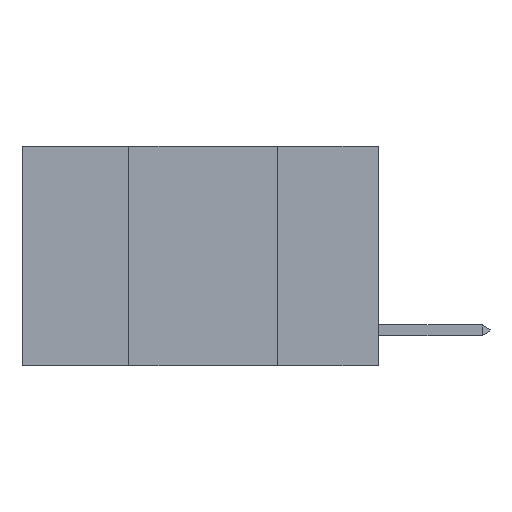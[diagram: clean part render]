
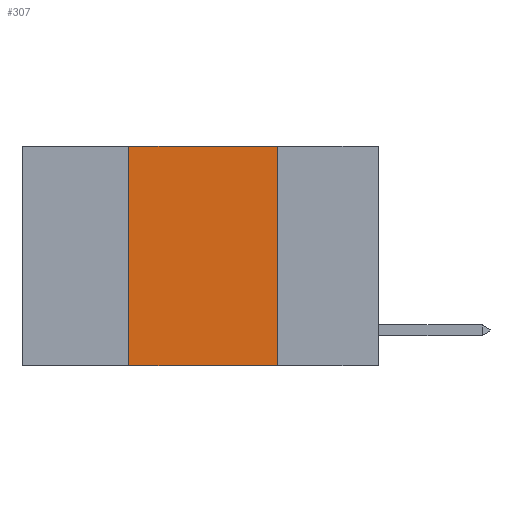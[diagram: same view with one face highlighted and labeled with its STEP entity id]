
A CAD part, left-side view. The second image highlights one B-rep face of the part: STEP entity #307.
In plain terms, the highlighted planar face has unit normal (-1, 0, 0).
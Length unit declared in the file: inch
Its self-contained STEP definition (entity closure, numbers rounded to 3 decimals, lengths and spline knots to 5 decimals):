
#183 = DIRECTION ( 'NONE',  ( 0., 0., 1. ) ) ;
#307 = ADVANCED_FACE ( 'NONE', ( #6110 ), #3378, .F. ) ;
#544 = DIRECTION ( 'NONE',  ( 0., 0., -1. ) ) ;
#657 = VERTEX_POINT ( 'NONE', #7695 ) ;
#913 = VERTEX_POINT ( 'NONE', #3167 ) ;
#953 = DIRECTION ( 'NONE',  ( 0., -1., 0. ) ) ;
#1651 = EDGE_CURVE ( 'NONE', #657, #3464, #7738, .T. ) ;
#1752 = LINE ( 'NONE', #4094, #5136 ) ;
#1923 = ORIENTED_EDGE ( 'NONE', *, *, #1651, .F. ) ;
#2455 = VECTOR ( 'NONE', #8177, 39.37008 ) ;
#2911 = ORIENTED_EDGE ( 'NONE', *, *, #6931, .F. ) ;
#3108 = CARTESIAN_POINT ( 'NONE',  ( 0., 0.42, 0. ) ) ;
#3167 = CARTESIAN_POINT ( 'NONE',  ( 0., 0.42, -0.37 ) ) ;
#3378 = PLANE ( 'NONE',  #3609 ) ;
#3464 = VERTEX_POINT ( 'NONE', #7201 ) ;
#3609 = AXIS2_PLACEMENT_3D ( 'NONE', #4952, #7891, #6412 ) ;
#3915 = CARTESIAN_POINT ( 'NONE',  ( 0., 0.17, -0.37 ) ) ;
#4050 = LINE ( 'NONE', #3108, #7164 ) ;
#4094 = CARTESIAN_POINT ( 'NONE',  ( 0., 0.17, 0. ) ) ;
#4255 = EDGE_CURVE ( 'NONE', #913, #657, #4050, .T. ) ;
#4435 = VECTOR ( 'NONE', #953, 39.37008 ) ;
#4569 = ORIENTED_EDGE ( 'NONE', *, *, #4255, .F. ) ;
#4868 = CARTESIAN_POINT ( 'NONE',  ( 0., 0.6, 0. ) ) ;
#4952 = CARTESIAN_POINT ( 'NONE',  ( 0., 0.6, 0. ) ) ;
#5050 = VERTEX_POINT ( 'NONE', #3915 ) ;
#5086 = ORIENTED_EDGE ( 'NONE', *, *, #5758, .T. ) ;
#5115 = EDGE_LOOP ( 'NONE', ( #2911, #1923, #4569, #5086 ) ) ;
#5136 = VECTOR ( 'NONE', #544, 39.37008 ) ;
#5758 = EDGE_CURVE ( 'NONE', #913, #5050, #6200, .T. ) ;
#6110 = FACE_OUTER_BOUND ( 'NONE', #5115, .T. ) ;
#6200 = LINE ( 'NONE', #7096, #4435 ) ;
#6412 = DIRECTION ( 'NONE',  ( 0., 0., -1. ) ) ;
#6931 = EDGE_CURVE ( 'NONE', #3464, #5050, #1752, .T. ) ;
#7096 = CARTESIAN_POINT ( 'NONE',  ( 0., 0.6, -0.37 ) ) ;
#7164 = VECTOR ( 'NONE', #183, 39.37008 ) ;
#7201 = CARTESIAN_POINT ( 'NONE',  ( 0., 0.17, 0. ) ) ;
#7695 = CARTESIAN_POINT ( 'NONE',  ( 0., 0.42, 0. ) ) ;
#7738 = LINE ( 'NONE', #4868, #2455 ) ;
#7891 = DIRECTION ( 'NONE',  ( 1., 0., 0. ) ) ;
#8177 = DIRECTION ( 'NONE',  ( 0., -1., 0. ) ) ;
